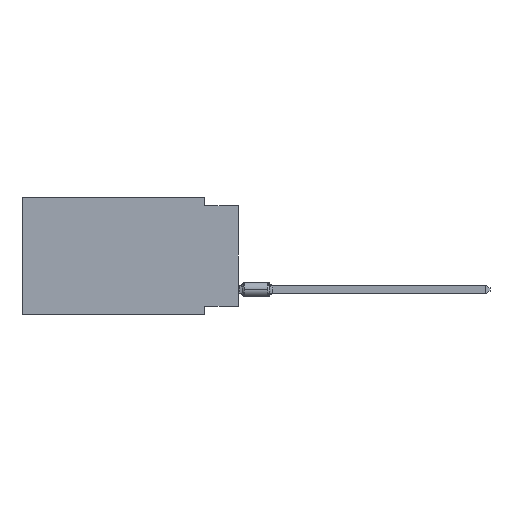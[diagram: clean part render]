
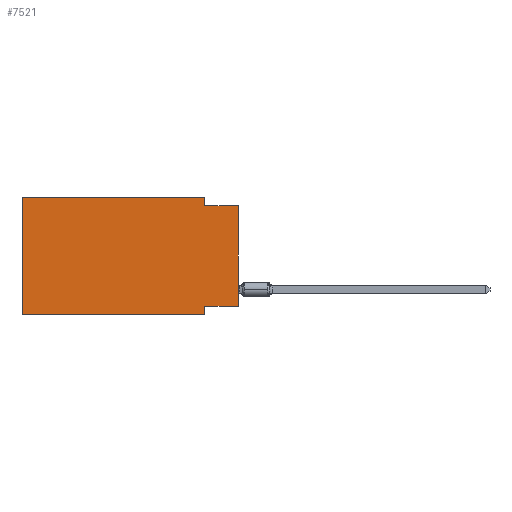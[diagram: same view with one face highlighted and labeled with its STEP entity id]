
A CAD part, left-side view. The second image highlights one B-rep face of the part: STEP entity #7521.
In plain terms, the highlighted planar face has unit normal (-1, 0, 0).
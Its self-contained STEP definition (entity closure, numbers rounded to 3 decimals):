
#896 = CARTESIAN_POINT ( 'NONE',  ( 0., 2.54, 0. ) ) ;
#1108 = CARTESIAN_POINT ( 'NONE',  ( 0., 0., -0.635 ) ) ;
#1222 = ORIENTED_EDGE ( 'NONE', *, *, #2162, .T. ) ;
#1394 = LINE ( 'NONE', #12792, #9789 ) ;
#1473 = DIRECTION ( 'NONE',  ( 0., 0., 1. ) ) ;
#1576 = EDGE_CURVE ( 'NONE', #6260, #6858, #1394, .T. ) ;
#2162 = EDGE_CURVE ( 'NONE', #11860, #8777, #15606, .T. ) ;
#2464 = EDGE_CURVE ( 'NONE', #14205, #15877, #7572, .T. ) ;
#2682 = CARTESIAN_POINT ( 'NONE',  ( 0., 2.54, 0. ) ) ;
#2753 = AXIS2_PLACEMENT_3D ( 'NONE', #8045, #13139, #15976 ) ;
#2918 = PLANE ( 'NONE',  #2753 ) ;
#2922 = CARTESIAN_POINT ( 'NONE',  ( 0., 2.54, -8.255 ) ) ;
#3829 = EDGE_CURVE ( 'NONE', #11860, #7051, #5874, .T. ) ;
#3941 = EDGE_LOOP ( 'NONE', ( #7016, #12312, #13397, #16046, #4115, #1222, #13318, #11879 ) ) ;
#4005 = VECTOR ( 'NONE', #6653, 1000. ) ;
#4115 = ORIENTED_EDGE ( 'NONE', *, *, #3829, .F. ) ;
#4425 = EDGE_CURVE ( 'NONE', #6260, #4942, #12994, .T. ) ;
#4608 = DIRECTION ( 'NONE',  ( 0., 0., 1. ) ) ;
#4781 = CARTESIAN_POINT ( 'NONE',  ( 0., 16.383, 0. ) ) ;
#4854 = CARTESIAN_POINT ( 'NONE',  ( 0., 0., -8.255 ) ) ;
#4942 = VERTEX_POINT ( 'NONE', #2922 ) ;
#5216 = DIRECTION ( 'NONE',  ( 0., 0., -1. ) ) ;
#5572 = CARTESIAN_POINT ( 'NONE',  ( 0., 0., -0.635 ) ) ;
#5874 = LINE ( 'NONE', #4781, #10940 ) ;
#6224 = DIRECTION ( 'NONE',  ( 0., -1., 0. ) ) ;
#6260 = VERTEX_POINT ( 'NONE', #4854 ) ;
#6266 = CARTESIAN_POINT ( 'NONE',  ( 0., 16.383, 0. ) ) ;
#6398 = VECTOR ( 'NONE', #11290, 1000. ) ;
#6558 = DIRECTION ( 'NONE',  ( 0., 1., 0. ) ) ;
#6653 = DIRECTION ( 'NONE',  ( 0., -1., 0. ) ) ;
#6858 = VERTEX_POINT ( 'NONE', #5572 ) ;
#6966 = VECTOR ( 'NONE', #7730, 1000. ) ;
#7016 = ORIENTED_EDGE ( 'NONE', *, *, #1576, .T. ) ;
#7051 = VERTEX_POINT ( 'NONE', #16273 ) ;
#7521 = ADVANCED_FACE ( 'NONE', ( #9297 ), #2918, .F. ) ;
#7572 = LINE ( 'NONE', #2682, #6966 ) ;
#7730 = DIRECTION ( 'NONE',  ( 0., 0., -1. ) ) ;
#8045 = CARTESIAN_POINT ( 'NONE',  ( 0., 16.383, 0. ) ) ;
#8507 = CARTESIAN_POINT ( 'NONE',  ( 0., 16.383, -8.89 ) ) ;
#8777 = VERTEX_POINT ( 'NONE', #15125 ) ;
#8868 = LINE ( 'NONE', #6266, #6398 ) ;
#9081 = CARTESIAN_POINT ( 'NONE',  ( 0., 0., -8.255 ) ) ;
#9297 = FACE_OUTER_BOUND ( 'NONE', #3941, .T. ) ;
#9345 = CARTESIAN_POINT ( 'NONE',  ( 0., 2.54, -0.635 ) ) ;
#9789 = VECTOR ( 'NONE', #1473, 1000. ) ;
#10262 = LINE ( 'NONE', #15356, #14062 ) ;
#10671 = CARTESIAN_POINT ( 'NONE',  ( 0., 16.383, -8.89 ) ) ;
#10940 = VECTOR ( 'NONE', #4608, 1000. ) ;
#11290 = DIRECTION ( 'NONE',  ( 0., -1., 0. ) ) ;
#11860 = VERTEX_POINT ( 'NONE', #8507 ) ;
#11879 = ORIENTED_EDGE ( 'NONE', *, *, #4425, .F. ) ;
#12312 = ORIENTED_EDGE ( 'NONE', *, *, #12402, .F. ) ;
#12402 = EDGE_CURVE ( 'NONE', #15877, #6858, #12586, .T. ) ;
#12455 = VECTOR ( 'NONE', #6224, 1000. ) ;
#12570 = VECTOR ( 'NONE', #6558, 1000. ) ;
#12586 = LINE ( 'NONE', #1108, #12455 ) ;
#12792 = CARTESIAN_POINT ( 'NONE',  ( 0., 0., 0. ) ) ;
#12994 = LINE ( 'NONE', #9081, #12570 ) ;
#13139 = DIRECTION ( 'NONE',  ( 1., 0., 0. ) ) ;
#13199 = EDGE_CURVE ( 'NONE', #4942, #8777, #10262, .T. ) ;
#13318 = ORIENTED_EDGE ( 'NONE', *, *, #13199, .F. ) ;
#13397 = ORIENTED_EDGE ( 'NONE', *, *, #2464, .F. ) ;
#14062 = VECTOR ( 'NONE', #5216, 1000. ) ;
#14205 = VERTEX_POINT ( 'NONE', #896 ) ;
#15125 = CARTESIAN_POINT ( 'NONE',  ( 0., 2.54, -8.89 ) ) ;
#15356 = CARTESIAN_POINT ( 'NONE',  ( 0., 2.54, -8.89 ) ) ;
#15606 = LINE ( 'NONE', #10671, #4005 ) ;
#15733 = EDGE_CURVE ( 'NONE', #7051, #14205, #8868, .T. ) ;
#15877 = VERTEX_POINT ( 'NONE', #9345 ) ;
#15976 = DIRECTION ( 'NONE',  ( 0., 0., -1. ) ) ;
#16046 = ORIENTED_EDGE ( 'NONE', *, *, #15733, .F. ) ;
#16273 = CARTESIAN_POINT ( 'NONE',  ( 0., 16.383, 0. ) ) ;
